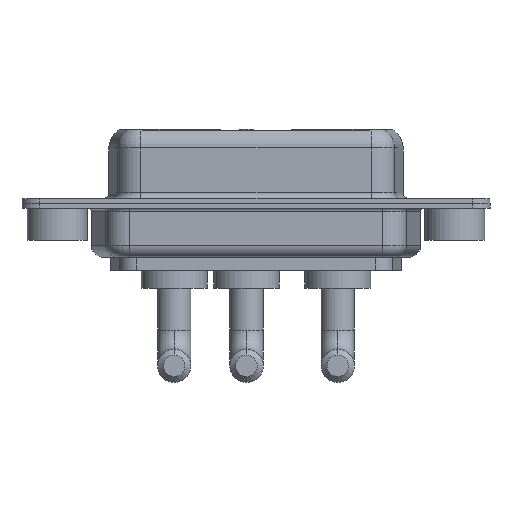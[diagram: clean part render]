
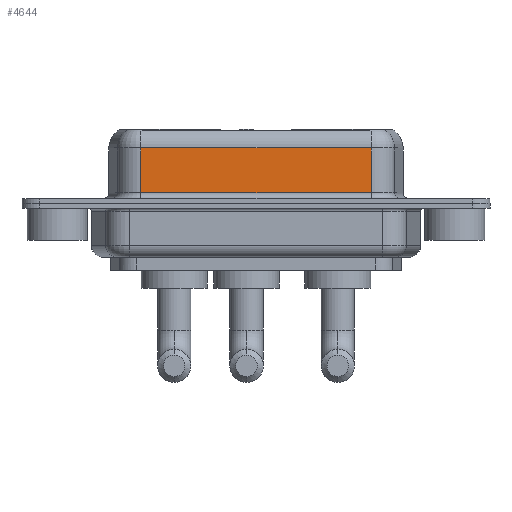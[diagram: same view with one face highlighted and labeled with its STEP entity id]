
A CAD part, front view. The second image highlights one B-rep face of the part: STEP entity #4644.
In plain terms, the highlighted planar face has unit normal (0, -1, 0).
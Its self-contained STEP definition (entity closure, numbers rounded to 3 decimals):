
#339 = LINE ( 'NONE', #11114, #6323 ) ;
#973 = VECTOR ( 'NONE', #10195, 1000. ) ;
#1133 = DIRECTION ( 'NONE',  ( -1., 0., 0. ) ) ;
#1608 = EDGE_CURVE ( 'NONE', #6233, #11412, #339, .T. ) ;
#1908 = AXIS2_PLACEMENT_3D ( 'NONE', #4460, #9810, #3279 ) ;
#2116 = EDGE_LOOP ( 'NONE', ( #3759, #11726, #12618, #10335 ) ) ;
#2279 = CARTESIAN_POINT ( 'NONE',  ( 26.287, -3.95, 6.4 ) ) ;
#3279 = DIRECTION ( 'NONE',  ( 0., 0., 1. ) ) ;
#3471 = CARTESIAN_POINT ( 'NONE',  ( 26.287, -3.95, 4.65 ) ) ;
#3759 = ORIENTED_EDGE ( 'NONE', *, *, #10698, .F. ) ;
#3816 = CARTESIAN_POINT ( 'NONE',  ( 7.013, -3.95, 4.65 ) ) ;
#4372 = DIRECTION ( 'NONE',  ( 0., 0., -1. ) ) ;
#4460 = CARTESIAN_POINT ( 'NONE',  ( 26.287, -3.95, 6.4 ) ) ;
#4644 = ADVANCED_FACE ( 'NONE', ( #7590 ), #5440, .F. ) ;
#4885 = VERTEX_POINT ( 'NONE', #5294 ) ;
#5294 = CARTESIAN_POINT ( 'NONE',  ( 26.287, -3.95, 0.9 ) ) ;
#5440 = PLANE ( 'NONE',  #1908 ) ;
#5596 = LINE ( 'NONE', #11980, #13176 ) ;
#5697 = VECTOR ( 'NONE', #4372, 1000. ) ;
#5705 = DIRECTION ( 'NONE',  ( 0., 0., -1. ) ) ;
#5902 = CARTESIAN_POINT ( 'NONE',  ( 26.287, -3.95, 0.9 ) ) ;
#6041 = VERTEX_POINT ( 'NONE', #3471 ) ;
#6233 = VERTEX_POINT ( 'NONE', #3816 ) ;
#6323 = VECTOR ( 'NONE', #5705, 1000. ) ;
#6435 = CARTESIAN_POINT ( 'NONE',  ( 7.013, -3.95, 0.9 ) ) ;
#7579 = EDGE_CURVE ( 'NONE', #6041, #6233, #5596, .T. ) ;
#7590 = FACE_OUTER_BOUND ( 'NONE', #2116, .T. ) ;
#8677 = LINE ( 'NONE', #2279, #5697 ) ;
#8769 = EDGE_CURVE ( 'NONE', #11412, #4885, #10258, .T. ) ;
#9810 = DIRECTION ( 'NONE',  ( 0., 1., 0. ) ) ;
#10195 = DIRECTION ( 'NONE',  ( 1., 0., 0. ) ) ;
#10258 = LINE ( 'NONE', #5902, #973 ) ;
#10335 = ORIENTED_EDGE ( 'NONE', *, *, #8769, .T. ) ;
#10698 = EDGE_CURVE ( 'NONE', #6041, #4885, #8677, .T. ) ;
#11114 = CARTESIAN_POINT ( 'NONE',  ( 7.013, -3.95, 6.4 ) ) ;
#11412 = VERTEX_POINT ( 'NONE', #6435 ) ;
#11726 = ORIENTED_EDGE ( 'NONE', *, *, #7579, .T. ) ;
#11980 = CARTESIAN_POINT ( 'NONE',  ( 26.287, -3.95, 4.65 ) ) ;
#12618 = ORIENTED_EDGE ( 'NONE', *, *, #1608, .T. ) ;
#13176 = VECTOR ( 'NONE', #1133, 1000. ) ;
